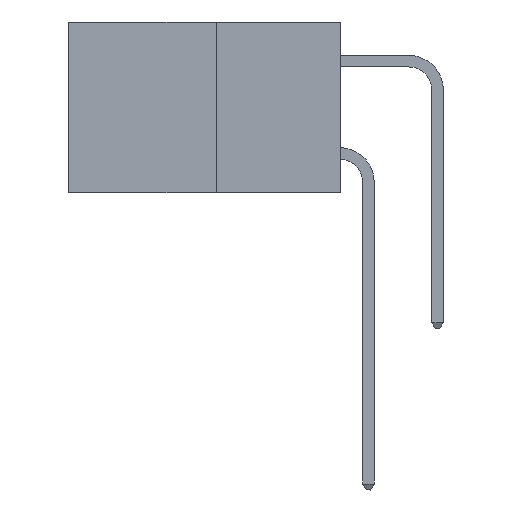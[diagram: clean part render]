
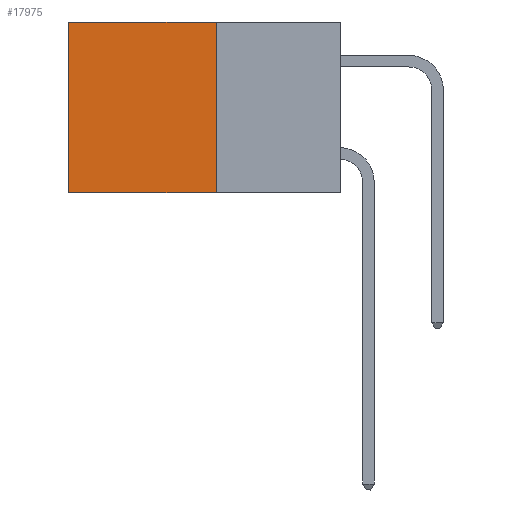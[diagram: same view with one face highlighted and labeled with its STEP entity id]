
A CAD part, left-side view. The second image highlights one B-rep face of the part: STEP entity #17975.
In plain terms, the highlighted planar face has unit normal (-1, 0, 0).
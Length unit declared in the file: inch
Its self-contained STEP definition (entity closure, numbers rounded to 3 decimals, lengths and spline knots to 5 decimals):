
#277 = CARTESIAN_POINT ( 'NONE',  ( 0.277, 0.59, -0.37 ) ) ;
#668 = VECTOR ( 'NONE', #20929, 39.37008 ) ;
#988 = VECTOR ( 'NONE', #25957, 39.37008 ) ;
#1152 = CARTESIAN_POINT ( 'NONE',  ( 0.277, 0.27, -0.37 ) ) ;
#1724 = PLANE ( 'NONE',  #11227 ) ;
#2053 = EDGE_CURVE ( 'NONE', #28255, #19643, #8959, .T. ) ;
#3536 = EDGE_CURVE ( 'NONE', #21038, #19643, #14973, .T. ) ;
#4889 = LINE ( 'NONE', #27698, #26279 ) ;
#7337 = DIRECTION ( 'NONE',  ( 1., 0., 0. ) ) ;
#8189 = DIRECTION ( 'NONE',  ( 0., 0., -1. ) ) ;
#8848 = DIRECTION ( 'NONE',  ( 0., 1., 0. ) ) ;
#8959 = LINE ( 'NONE', #20766, #668 ) ;
#11227 = AXIS2_PLACEMENT_3D ( 'NONE', #24067, #7337, #26872 ) ;
#13264 = EDGE_CURVE ( 'NONE', #26148, #28255, #28523, .T. ) ;
#13716 = VECTOR ( 'NONE', #8848, 39.37008 ) ;
#14193 = CARTESIAN_POINT ( 'NONE',  ( 0.277, 0.27, 0. ) ) ;
#14973 = LINE ( 'NONE', #1152, #988 ) ;
#15708 = ORIENTED_EDGE ( 'NONE', *, *, #13264, .T. ) ;
#16057 = ORIENTED_EDGE ( 'NONE', *, *, #3536, .F. ) ;
#17164 = CARTESIAN_POINT ( 'NONE',  ( 0.277, 0.27, 0. ) ) ;
#17975 = ADVANCED_FACE ( 'NONE', ( #32161 ), #1724, .F. ) ;
#19643 = VERTEX_POINT ( 'NONE', #277 ) ;
#20633 = EDGE_CURVE ( 'NONE', #26148, #21038, #4889, .T. ) ;
#20766 = CARTESIAN_POINT ( 'NONE',  ( 0.277, 0.59, -0.37 ) ) ;
#20929 = DIRECTION ( 'NONE',  ( 0., 0., -1. ) ) ;
#20971 = CARTESIAN_POINT ( 'NONE',  ( 0.277, 0.27, -0.37 ) ) ;
#21038 = VERTEX_POINT ( 'NONE', #20971 ) ;
#23034 = CARTESIAN_POINT ( 'NONE',  ( 0.277, 0.59, 0. ) ) ;
#24067 = CARTESIAN_POINT ( 'NONE',  ( 0.277, 0.27, -0.37 ) ) ;
#25957 = DIRECTION ( 'NONE',  ( 0., 1., 0. ) ) ;
#26148 = VERTEX_POINT ( 'NONE', #14193 ) ;
#26279 = VECTOR ( 'NONE', #8189, 39.37008 ) ;
#26872 = DIRECTION ( 'NONE',  ( 0., 0., -1. ) ) ;
#27698 = CARTESIAN_POINT ( 'NONE',  ( 0.277, 0.27, -0.37 ) ) ;
#28255 = VERTEX_POINT ( 'NONE', #23034 ) ;
#28266 = EDGE_LOOP ( 'NONE', ( #33733, #16057, #28771, #15708 ) ) ;
#28523 = LINE ( 'NONE', #17164, #13716 ) ;
#28771 = ORIENTED_EDGE ( 'NONE', *, *, #20633, .F. ) ;
#32161 = FACE_OUTER_BOUND ( 'NONE', #28266, .T. ) ;
#33733 = ORIENTED_EDGE ( 'NONE', *, *, #2053, .T. ) ;
